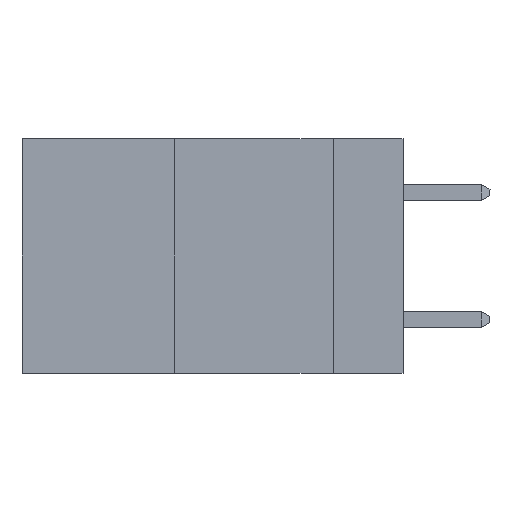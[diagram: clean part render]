
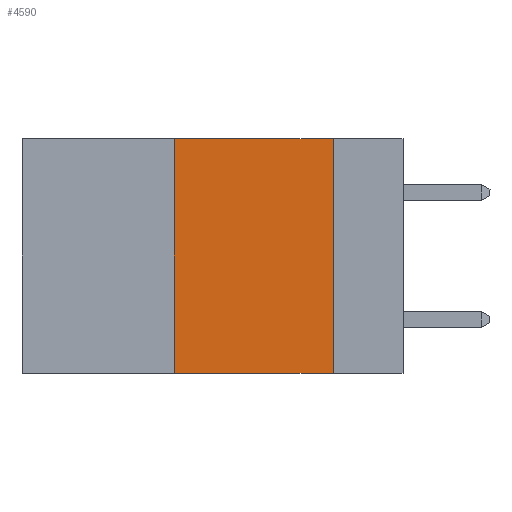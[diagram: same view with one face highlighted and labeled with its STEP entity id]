
A CAD part, left-side view. The second image highlights one B-rep face of the part: STEP entity #4590.
In plain terms, the highlighted planar face has unit normal (-1, 0, 0).
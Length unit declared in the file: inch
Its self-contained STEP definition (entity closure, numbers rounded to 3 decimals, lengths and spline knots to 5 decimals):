
#136 = CARTESIAN_POINT ( 'NONE',  ( 0., 0.11, 0. ) ) ;
#560 = VERTEX_POINT ( 'NONE', #7364 ) ;
#798 = CARTESIAN_POINT ( 'NONE',  ( 0., 0.6, -0.37 ) ) ;
#1331 = ORIENTED_EDGE ( 'NONE', *, *, #9907, .F. ) ;
#1546 = CARTESIAN_POINT ( 'NONE',  ( 0., 0.6, 0. ) ) ;
#1779 = VERTEX_POINT ( 'NONE', #136 ) ;
#1786 = DIRECTION ( 'NONE',  ( 0., -1., 0. ) ) ;
#2142 = EDGE_LOOP ( 'NONE', ( #10292, #9839, #1331, #5521 ) ) ;
#3285 = VECTOR ( 'NONE', #4178, 39.37008 ) ;
#3625 = VECTOR ( 'NONE', #4960, 39.37008 ) ;
#4178 = DIRECTION ( 'NONE',  ( 0., -1., 0. ) ) ;
#4391 = VECTOR ( 'NONE', #8904, 39.37008 ) ;
#4590 = ADVANCED_FACE ( 'NONE', ( #10110 ), #7866, .F. ) ;
#4678 = EDGE_CURVE ( 'NONE', #10409, #1779, #8248, .T. ) ;
#4695 = VECTOR ( 'NONE', #1786, 39.37008 ) ;
#4960 = DIRECTION ( 'NONE',  ( 0., 0., -1. ) ) ;
#5092 = CARTESIAN_POINT ( 'NONE',  ( 0., 0.11, -0.37 ) ) ;
#5294 = CARTESIAN_POINT ( 'NONE',  ( 0., 0.6, 0. ) ) ;
#5372 = DIRECTION ( 'NONE',  ( 1., 0., 0. ) ) ;
#5521 = ORIENTED_EDGE ( 'NONE', *, *, #10128, .T. ) ;
#5556 = CARTESIAN_POINT ( 'NONE',  ( 0., 0.36, 0. ) ) ;
#6643 = LINE ( 'NONE', #5556, #4391 ) ;
#6709 = LINE ( 'NONE', #798, #4695 ) ;
#6927 = CARTESIAN_POINT ( 'NONE',  ( 0., 0.36, 0. ) ) ;
#7032 = LINE ( 'NONE', #9215, #3625 ) ;
#7109 = EDGE_CURVE ( 'NONE', #1779, #10800, #7032, .T. ) ;
#7364 = CARTESIAN_POINT ( 'NONE',  ( 0., 0.36, -0.37 ) ) ;
#7866 = PLANE ( 'NONE',  #8975 ) ;
#8248 = LINE ( 'NONE', #1546, #3285 ) ;
#8904 = DIRECTION ( 'NONE',  ( 0., 0., 1. ) ) ;
#8975 = AXIS2_PLACEMENT_3D ( 'NONE', #5294, #5372, #9606 ) ;
#9215 = CARTESIAN_POINT ( 'NONE',  ( 0., 0.11, 0. ) ) ;
#9606 = DIRECTION ( 'NONE',  ( 0., 0., -1. ) ) ;
#9839 = ORIENTED_EDGE ( 'NONE', *, *, #4678, .F. ) ;
#9907 = EDGE_CURVE ( 'NONE', #560, #10409, #6643, .T. ) ;
#10110 = FACE_OUTER_BOUND ( 'NONE', #2142, .T. ) ;
#10128 = EDGE_CURVE ( 'NONE', #560, #10800, #6709, .T. ) ;
#10292 = ORIENTED_EDGE ( 'NONE', *, *, #7109, .F. ) ;
#10409 = VERTEX_POINT ( 'NONE', #6927 ) ;
#10800 = VERTEX_POINT ( 'NONE', #5092 ) ;
